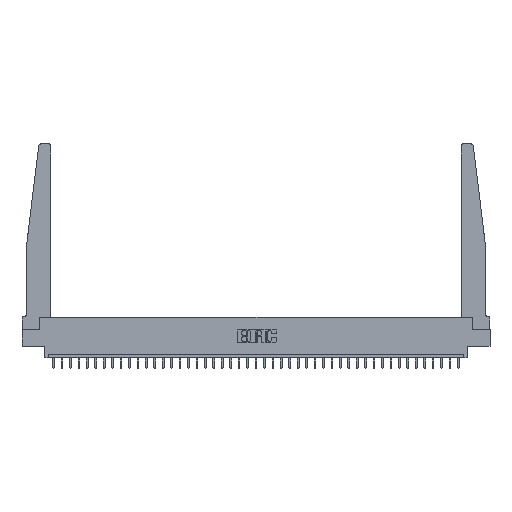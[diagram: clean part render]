
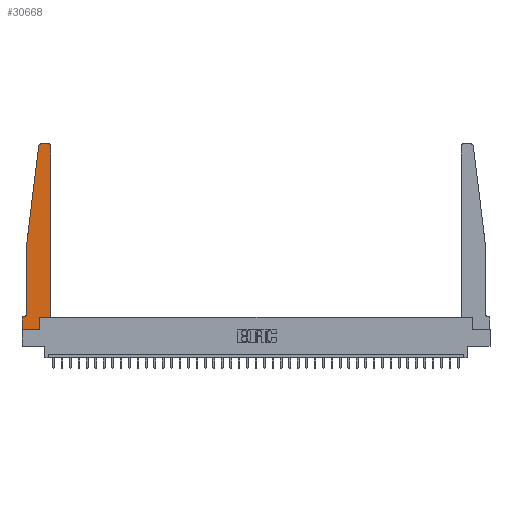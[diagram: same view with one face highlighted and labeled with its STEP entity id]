
A CAD part, top view. The second image highlights one B-rep face of the part: STEP entity #30668.
In plain terms, the highlighted planar face has unit normal (0, 0, 1).
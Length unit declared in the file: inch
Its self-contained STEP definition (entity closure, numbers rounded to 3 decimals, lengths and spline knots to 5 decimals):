
#191 = EDGE_CURVE ( 'NONE', #21984, #11332, #27391, .T. ) ;
#312 = VECTOR ( 'NONE', #11261, 39.37008 ) ;
#329 = AXIS2_PLACEMENT_3D ( 'NONE', #3207, #32177, #10846 ) ;
#752 = ORIENTED_EDGE ( 'NONE', *, *, #31081, .T. ) ;
#774 = EDGE_CURVE ( 'NONE', #24125, #28329, #8677, .T. ) ;
#829 = DIRECTION ( 'NONE',  ( -1., 0., 0. ) ) ;
#1402 = CARTESIAN_POINT ( 'NONE',  ( 0., 0., 0.37 ) ) ;
#1948 = CARTESIAN_POINT ( 'NONE',  ( 0.27653, 2.72, 0.37 ) ) ;
#2152 = CARTESIAN_POINT ( 'NONE',  ( 0.395, 2.75, 0.37 ) ) ;
#2160 = ORIENTED_EDGE ( 'NONE', *, *, #774, .T. ) ;
#2248 = AXIS2_PLACEMENT_3D ( 'NONE', #1948, #10328, #12746 ) ;
#2583 = EDGE_LOOP ( 'NONE', ( #11183, #6220, #752, #2160, #18020, #24143, #33288, #6087, #17781, #24976, #8887, #23216 ) ) ;
#2719 = CARTESIAN_POINT ( 'NONE',  ( 0.065, 1.25, 0.37 ) ) ;
#3089 = LINE ( 'NONE', #6215, #5595 ) ;
#3207 = CARTESIAN_POINT ( 'NONE',  ( 0.395, 2.72, 0.37 ) ) ;
#4120 = VERTEX_POINT ( 'NONE', #15381 ) ;
#4266 = DIRECTION ( 'NONE',  ( -1., 0., 0. ) ) ;
#4589 = CARTESIAN_POINT ( 'NONE',  ( 0.27653, 2.75, 0.37 ) ) ;
#4611 = CARTESIAN_POINT ( 'NONE',  ( 0., 0.1875, 0.37 ) ) ;
#4861 = VECTOR ( 'NONE', #16053, 39.37008 ) ;
#5178 = VECTOR ( 'NONE', #29859, 39.37008 ) ;
#5595 = VECTOR ( 'NONE', #14056, 39.37008 ) ;
#6087 = ORIENTED_EDGE ( 'NONE', *, *, #191, .T. ) ;
#6215 = CARTESIAN_POINT ( 'NONE',  ( 0.065, 1.25, 0.37 ) ) ;
#6220 = ORIENTED_EDGE ( 'NONE', *, *, #15775, .T. ) ;
#6821 = LINE ( 'NONE', #29519, #5178 ) ;
#7205 = CARTESIAN_POINT ( 'NONE',  ( 0.065, 0.1875, 0.37 ) ) ;
#8121 = CARTESIAN_POINT ( 'NONE',  ( 0., 0., 0.37 ) ) ;
#8467 = CARTESIAN_POINT ( 'NONE',  ( 0.2605, 0.18, 0.37 ) ) ;
#8591 = LINE ( 'NONE', #29813, #4861 ) ;
#8677 = LINE ( 'NONE', #2719, #23611 ) ;
#8887 = ORIENTED_EDGE ( 'NONE', *, *, #34090, .T. ) ;
#9190 = EDGE_CURVE ( 'NONE', #20263, #19362, #6821, .T. ) ;
#9943 = CARTESIAN_POINT ( 'NONE',  ( 0.25, 2.75, 0.37 ) ) ;
#10328 = DIRECTION ( 'NONE',  ( 0., 0., 1. ) ) ;
#10846 = DIRECTION ( 'NONE',  ( 1., 0., 0. ) ) ;
#11043 = CARTESIAN_POINT ( 'NONE',  ( 0., 0., 0.37 ) ) ;
#11183 = ORIENTED_EDGE ( 'NONE', *, *, #16652, .T. ) ;
#11261 = DIRECTION ( 'NONE',  ( 0., -1., 0. ) ) ;
#11332 = VERTEX_POINT ( 'NONE', #13284 ) ;
#12746 = DIRECTION ( 'NONE',  ( 1., 0., 0. ) ) ;
#12991 = LINE ( 'NONE', #9943, #33327 ) ;
#13284 = CARTESIAN_POINT ( 'NONE',  ( 0.2605, 0., 0.37 ) ) ;
#14056 = DIRECTION ( 'NONE',  ( -0.122, -0.992, 0. ) ) ;
#14264 = CARTESIAN_POINT ( 'NONE',  ( 0.015, 0.2375, 0.37 ) ) ;
#15189 = VERTEX_POINT ( 'NONE', #30277 ) ;
#15279 = CARTESIAN_POINT ( 'NONE',  ( 0.2605, 0.18, 0.37 ) ) ;
#15381 = CARTESIAN_POINT ( 'NONE',  ( 0.24675, 2.72367, 0.37 ) ) ;
#15769 = EDGE_CURVE ( 'NONE', #15189, #31515, #22589, .T. ) ;
#15775 = EDGE_CURVE ( 'NONE', #21475, #4120, #18377, .T. ) ;
#15999 = VERTEX_POINT ( 'NONE', #2152 ) ;
#16053 = DIRECTION ( 'NONE',  ( 0., 1., 0. ) ) ;
#16652 = EDGE_CURVE ( 'NONE', #15999, #21475, #12991, .T. ) ;
#17063 = EDGE_CURVE ( 'NONE', #11332, #20263, #32036, .T. ) ;
#17768 = VERTEX_POINT ( 'NONE', #18498 ) ;
#17781 = ORIENTED_EDGE ( 'NONE', *, *, #17063, .T. ) ;
#17858 = AXIS2_PLACEMENT_3D ( 'NONE', #4611, #20486, #23384 ) ;
#18020 = ORIENTED_EDGE ( 'NONE', *, *, #25187, .T. ) ;
#18232 = VECTOR ( 'NONE', #34198, 39.37008 ) ;
#18377 = CIRCLE ( 'NONE', #2248, 0.03 ) ;
#18498 = CARTESIAN_POINT ( 'NONE',  ( 0.425, 2.72, 0.37 ) ) ;
#19216 = DIRECTION ( 'NONE',  ( 0., 1., 0. ) ) ;
#19362 = VERTEX_POINT ( 'NONE', #27127 ) ;
#20263 = VERTEX_POINT ( 'NONE', #15279 ) ;
#20486 = DIRECTION ( 'NONE',  ( 0., 0., 1. ) ) ;
#20792 = EDGE_CURVE ( 'NONE', #17768, #15999, #25387, .T. ) ;
#20945 = VECTOR ( 'NONE', #25778, 39.37008 ) ;
#21475 = VERTEX_POINT ( 'NONE', #4589 ) ;
#21984 = VERTEX_POINT ( 'NONE', #1402 ) ;
#22589 = LINE ( 'NONE', #7205, #20945 ) ;
#23216 = ORIENTED_EDGE ( 'NONE', *, *, #20792, .T. ) ;
#23384 = DIRECTION ( 'NONE',  ( 1., 0., 0. ) ) ;
#23611 = VECTOR ( 'NONE', #28943, 39.37008 ) ;
#23694 = CARTESIAN_POINT ( 'NONE',  ( 0., 0.1875, 0.37 ) ) ;
#23735 = VECTOR ( 'NONE', #19216, 39.37008 ) ;
#24120 = EDGE_CURVE ( 'NONE', #31515, #21984, #32693, .T. ) ;
#24125 = VERTEX_POINT ( 'NONE', #27064 ) ;
#24143 = ORIENTED_EDGE ( 'NONE', *, *, #15769, .T. ) ;
#24976 = ORIENTED_EDGE ( 'NONE', *, *, #9190, .T. ) ;
#25187 = EDGE_CURVE ( 'NONE', #28329, #15189, #28710, .T. ) ;
#25387 = CIRCLE ( 'NONE', #329, 0.03 ) ;
#25574 = CARTESIAN_POINT ( 'NONE',  ( 0.065, 0.2375, 0.37 ) ) ;
#25778 = DIRECTION ( 'NONE',  ( -1., 0., 0. ) ) ;
#27064 = CARTESIAN_POINT ( 'NONE',  ( 0.065, 1.25, 0.37 ) ) ;
#27127 = CARTESIAN_POINT ( 'NONE',  ( 0.425, 0.18, 0.37 ) ) ;
#27391 = LINE ( 'NONE', #8121, #18232 ) ;
#27983 = AXIS2_PLACEMENT_3D ( 'NONE', #14264, #29930, #829 ) ;
#28329 = VERTEX_POINT ( 'NONE', #25574 ) ;
#28710 = CIRCLE ( 'NONE', #27983, 0.05 ) ;
#28943 = DIRECTION ( 'NONE',  ( 0., -1., 0. ) ) ;
#29519 = CARTESIAN_POINT ( 'NONE',  ( 0.425, 0.18, 0.37 ) ) ;
#29813 = CARTESIAN_POINT ( 'NONE',  ( 0.425, 0.18, 0.37 ) ) ;
#29859 = DIRECTION ( 'NONE',  ( 1., 0., 0. ) ) ;
#29930 = DIRECTION ( 'NONE',  ( 0., 0., -1. ) ) ;
#30277 = CARTESIAN_POINT ( 'NONE',  ( 0.015, 0.1875, 0.37 ) ) ;
#30668 = ADVANCED_FACE ( 'NONE', ( #33354 ), #30918, .T. ) ;
#30918 = PLANE ( 'NONE',  #17858 ) ;
#31081 = EDGE_CURVE ( 'NONE', #4120, #24125, #3089, .T. ) ;
#31515 = VERTEX_POINT ( 'NONE', #23694 ) ;
#32036 = LINE ( 'NONE', #8467, #23735 ) ;
#32177 = DIRECTION ( 'NONE',  ( 0., 0., 1. ) ) ;
#32693 = LINE ( 'NONE', #11043, #312 ) ;
#33288 = ORIENTED_EDGE ( 'NONE', *, *, #24120, .T. ) ;
#33327 = VECTOR ( 'NONE', #4266, 39.37008 ) ;
#33354 = FACE_OUTER_BOUND ( 'NONE', #2583, .T. ) ;
#34090 = EDGE_CURVE ( 'NONE', #19362, #17768, #8591, .T. ) ;
#34198 = DIRECTION ( 'NONE',  ( 1., 0., 0. ) ) ;
